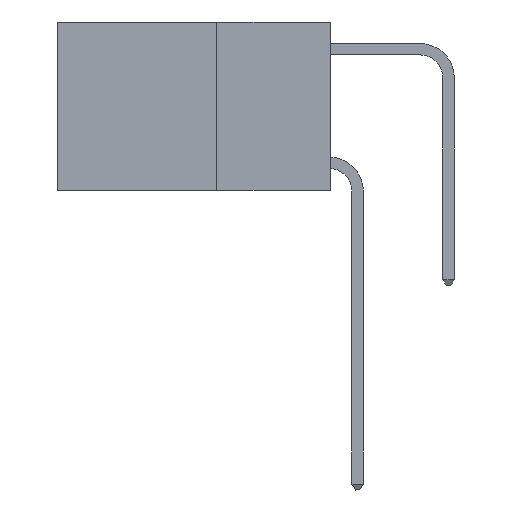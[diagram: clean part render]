
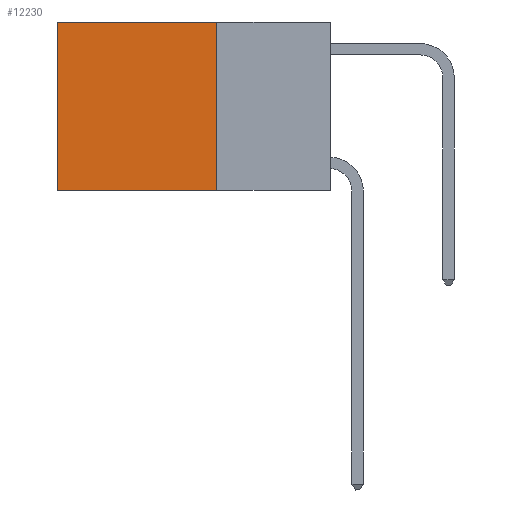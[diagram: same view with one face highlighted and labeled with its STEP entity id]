
A CAD part, left-side view. The second image highlights one B-rep face of the part: STEP entity #12230.
In plain terms, the highlighted planar face has unit normal (-1, 0, 0).
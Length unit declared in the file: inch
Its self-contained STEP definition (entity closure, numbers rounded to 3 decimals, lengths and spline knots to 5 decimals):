
#1414 = ORIENTED_EDGE ( 'NONE', *, *, #3025, .F. ) ;
#1846 = VERTEX_POINT ( 'NONE', #2529 ) ;
#1942 = VECTOR ( 'NONE', #10850, 39.37008 ) ;
#2529 = CARTESIAN_POINT ( 'NONE',  ( 0.2625, 0.6, 0. ) ) ;
#2919 = VECTOR ( 'NONE', #19014, 39.37008 ) ;
#3025 = EDGE_CURVE ( 'NONE', #20996, #16268, #19389, .T. ) ;
#3606 = LINE ( 'NONE', #14563, #2919 ) ;
#5446 = AXIS2_PLACEMENT_3D ( 'NONE', #21718, #8697, #23906 ) ;
#5771 = EDGE_CURVE ( 'NONE', #10971, #20996, #20955, .T. ) ;
#6924 = CARTESIAN_POINT ( 'NONE',  ( 0.2625, 0.25, 0. ) ) ;
#8627 = CARTESIAN_POINT ( 'NONE',  ( 0.2625, 0.25, -0.37 ) ) ;
#8697 = DIRECTION ( 'NONE',  ( 1., 0., 0. ) ) ;
#9148 = DIRECTION ( 'NONE',  ( 0., 0., -1. ) ) ;
#10850 = DIRECTION ( 'NONE',  ( 0., 1., 0. ) ) ;
#10971 = VERTEX_POINT ( 'NONE', #15633 ) ;
#11753 = EDGE_LOOP ( 'NONE', ( #13911, #1414, #17261, #16951 ) ) ;
#11946 = DIRECTION ( 'NONE',  ( 0., 1., 0. ) ) ;
#12230 = ADVANCED_FACE ( 'NONE', ( #19338 ), #12944, .F. ) ;
#12944 = PLANE ( 'NONE',  #5446 ) ;
#13911 = ORIENTED_EDGE ( 'NONE', *, *, #21862, .T. ) ;
#14563 = CARTESIAN_POINT ( 'NONE',  ( 0.2625, 0.6, 0. ) ) ;
#15633 = CARTESIAN_POINT ( 'NONE',  ( 0.2625, 0.25, 0. ) ) ;
#16268 = VERTEX_POINT ( 'NONE', #22414 ) ;
#16951 = ORIENTED_EDGE ( 'NONE', *, *, #24110, .T. ) ;
#17261 = ORIENTED_EDGE ( 'NONE', *, *, #5771, .F. ) ;
#19014 = DIRECTION ( 'NONE',  ( 0., 0., -1. ) ) ;
#19338 = FACE_OUTER_BOUND ( 'NONE', #11753, .T. ) ;
#19389 = LINE ( 'NONE', #8627, #1942 ) ;
#20270 = VECTOR ( 'NONE', #9148, 39.37008 ) ;
#20887 = LINE ( 'NONE', #27044, #25947 ) ;
#20955 = LINE ( 'NONE', #6924, #20270 ) ;
#20996 = VERTEX_POINT ( 'NONE', #26594 ) ;
#21718 = CARTESIAN_POINT ( 'NONE',  ( 0.2625, 0.25, 0. ) ) ;
#21862 = EDGE_CURVE ( 'NONE', #1846, #16268, #3606, .T. ) ;
#22414 = CARTESIAN_POINT ( 'NONE',  ( 0.2625, 0.6, -0.37 ) ) ;
#23906 = DIRECTION ( 'NONE',  ( 0., 0., -1. ) ) ;
#24110 = EDGE_CURVE ( 'NONE', #10971, #1846, #20887, .T. ) ;
#25947 = VECTOR ( 'NONE', #11946, 39.37008 ) ;
#26594 = CARTESIAN_POINT ( 'NONE',  ( 0.2625, 0.25, -0.37 ) ) ;
#27044 = CARTESIAN_POINT ( 'NONE',  ( 0.2625, 0.25, 0. ) ) ;
